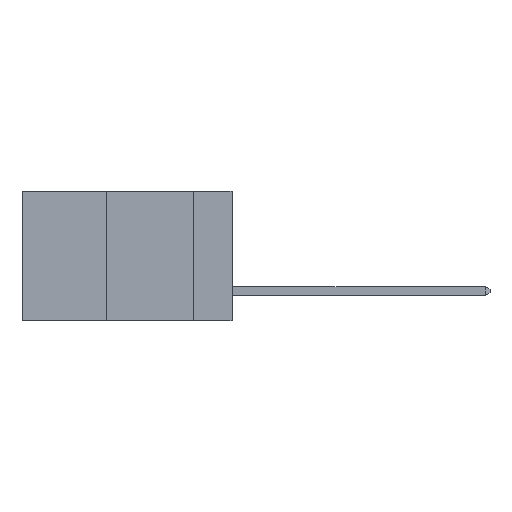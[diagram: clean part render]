
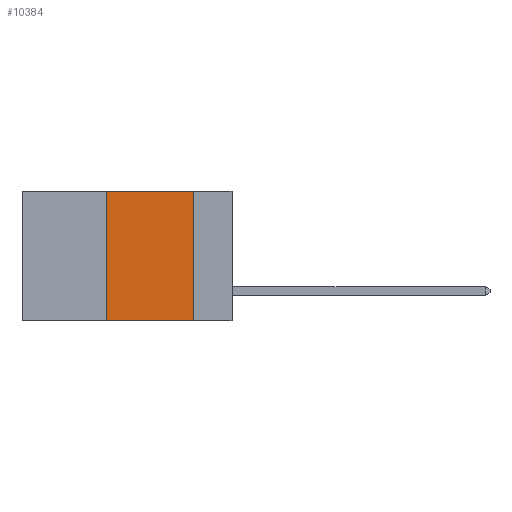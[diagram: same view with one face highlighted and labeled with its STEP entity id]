
A CAD part, left-side view. The second image highlights one B-rep face of the part: STEP entity #10384.
In plain terms, the highlighted planar face has unit normal (-1, 0, 0).
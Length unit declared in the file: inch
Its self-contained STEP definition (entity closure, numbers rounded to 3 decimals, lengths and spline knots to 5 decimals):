
#198 = LINE ( 'NONE', #3031, #9213 ) ;
#256 = DIRECTION ( 'NONE',  ( 0., 0., -1. ) ) ;
#357 = CARTESIAN_POINT ( 'NONE',  ( 0., 0.6, 0. ) ) ;
#639 = LINE ( 'NONE', #4465, #5087 ) ;
#690 = VECTOR ( 'NONE', #2245, 39.37008 ) ;
#838 = VERTEX_POINT ( 'NONE', #2710 ) ;
#873 = EDGE_CURVE ( 'NONE', #3192, #9489, #639, .T. ) ;
#1564 = VECTOR ( 'NONE', #8288, 39.37008 ) ;
#1954 = CARTESIAN_POINT ( 'NONE',  ( 0., 0.11, 0. ) ) ;
#2245 = DIRECTION ( 'NONE',  ( 0., 0., 1. ) ) ;
#2290 = FACE_OUTER_BOUND ( 'NONE', #9267, .T. ) ;
#2350 = EDGE_CURVE ( 'NONE', #7553, #9489, #198, .T. ) ;
#2710 = CARTESIAN_POINT ( 'NONE',  ( 0., 0.36, 0. ) ) ;
#3031 = CARTESIAN_POINT ( 'NONE',  ( 0., 0.6, -0.37 ) ) ;
#3192 = VERTEX_POINT ( 'NONE', #1954 ) ;
#3378 = LINE ( 'NONE', #9094, #690 ) ;
#4465 = CARTESIAN_POINT ( 'NONE',  ( 0., 0.11, 0. ) ) ;
#4699 = DIRECTION ( 'NONE',  ( 0., -1., 0. ) ) ;
#4948 = DIRECTION ( 'NONE',  ( 0., 0., -1. ) ) ;
#4987 = CARTESIAN_POINT ( 'NONE',  ( 0., 0.11, -0.37 ) ) ;
#5087 = VECTOR ( 'NONE', #4948, 39.37008 ) ;
#5410 = CARTESIAN_POINT ( 'NONE',  ( 0., 0.36, -0.37 ) ) ;
#5585 = DIRECTION ( 'NONE',  ( 1., 0., 0. ) ) ;
#5822 = EDGE_CURVE ( 'NONE', #7553, #838, #3378, .T. ) ;
#5999 = ORIENTED_EDGE ( 'NONE', *, *, #873, .F. ) ;
#7324 = PLANE ( 'NONE',  #8233 ) ;
#7553 = VERTEX_POINT ( 'NONE', #5410 ) ;
#8233 = AXIS2_PLACEMENT_3D ( 'NONE', #10550, #5585, #256 ) ;
#8288 = DIRECTION ( 'NONE',  ( 0., -1., 0. ) ) ;
#8461 = LINE ( 'NONE', #357, #1564 ) ;
#9094 = CARTESIAN_POINT ( 'NONE',  ( 0., 0.36, 0. ) ) ;
#9211 = ORIENTED_EDGE ( 'NONE', *, *, #5822, .F. ) ;
#9213 = VECTOR ( 'NONE', #4699, 39.37008 ) ;
#9267 = EDGE_LOOP ( 'NONE', ( #5999, #9320, #9211, #10345 ) ) ;
#9320 = ORIENTED_EDGE ( 'NONE', *, *, #11120, .F. ) ;
#9489 = VERTEX_POINT ( 'NONE', #4987 ) ;
#10345 = ORIENTED_EDGE ( 'NONE', *, *, #2350, .T. ) ;
#10384 = ADVANCED_FACE ( 'NONE', ( #2290 ), #7324, .F. ) ;
#10550 = CARTESIAN_POINT ( 'NONE',  ( 0., 0.6, 0. ) ) ;
#11120 = EDGE_CURVE ( 'NONE', #838, #3192, #8461, .T. ) ;
